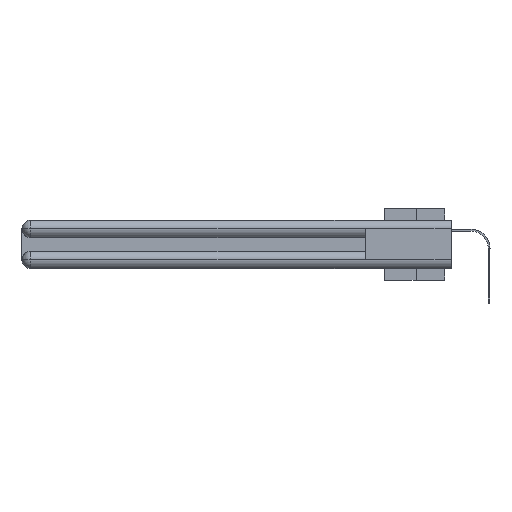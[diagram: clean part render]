
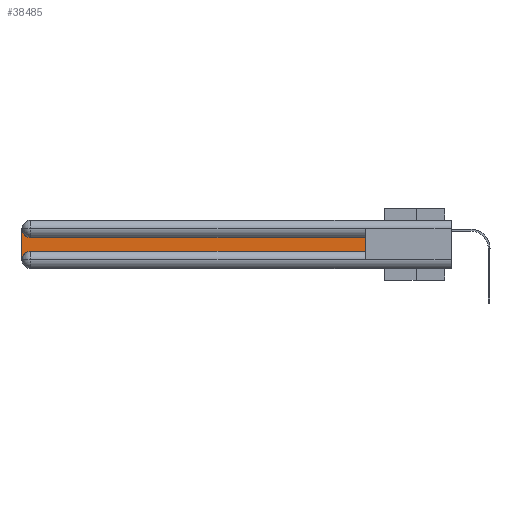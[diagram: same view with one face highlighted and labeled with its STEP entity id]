
A CAD part, left-side view. The second image highlights one B-rep face of the part: STEP entity #38485.
In plain terms, the highlighted planar face has unit normal (-1, 0, 0).
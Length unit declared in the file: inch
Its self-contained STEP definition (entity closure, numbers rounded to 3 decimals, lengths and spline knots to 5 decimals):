
#210 = DIRECTION ( 'NONE',  ( 1., 0., 0. ) ) ;
#868 = CARTESIAN_POINT ( 'NONE',  ( 0.075, 3., -0.0625 ) ) ;
#1109 = CARTESIAN_POINT ( 'NONE',  ( 0.075, 0.6, -0.2175 ) ) ;
#1456 = DIRECTION ( 'NONE',  ( 0., 0., 1. ) ) ;
#1462 = EDGE_CURVE ( 'NONE', #36980, #13549, #33551, .T. ) ;
#2479 = CARTESIAN_POINT ( 'NONE',  ( 0.075, 3., -0.2175 ) ) ;
#2937 = CARTESIAN_POINT ( 'NONE',  ( 0.075, 0.6, -0.1225 ) ) ;
#4326 = VECTOR ( 'NONE', #6533, 39.37008 ) ;
#5274 = ORIENTED_EDGE ( 'NONE', *, *, #5293, .T. ) ;
#5293 = EDGE_CURVE ( 'NONE', #35049, #37860, #30685, .T. ) ;
#5559 = LINE ( 'NONE', #17542, #23893 ) ;
#6024 = AXIS2_PLACEMENT_3D ( 'NONE', #17733, #10886, #17164 ) ;
#6533 = DIRECTION ( 'NONE',  ( 0., -1., 0. ) ) ;
#7232 = EDGE_CURVE ( 'NONE', #13549, #35049, #35408, .T. ) ;
#7799 = EDGE_CURVE ( 'NONE', #11284, #36980, #5559, .T. ) ;
#8370 = DIRECTION ( 'NONE',  ( 1., 0., 0. ) ) ;
#9089 = EDGE_CURVE ( 'NONE', #37860, #21161, #32810, .T. ) ;
#10886 = DIRECTION ( 'NONE',  ( 1., 0., 0. ) ) ;
#11266 = CARTESIAN_POINT ( 'NONE',  ( 0.075, 3., -0.2775 ) ) ;
#11284 = VERTEX_POINT ( 'NONE', #2937 ) ;
#11305 = FACE_OUTER_BOUND ( 'NONE', #34375, .T. ) ;
#13052 = ORIENTED_EDGE ( 'NONE', *, *, #7799, .T. ) ;
#13549 = VERTEX_POINT ( 'NONE', #868 ) ;
#13757 = EDGE_CURVE ( 'NONE', #21161, #11284, #31822, .T. ) ;
#14401 = DIRECTION ( 'NONE',  ( 0., 1., 0. ) ) ;
#15735 = VECTOR ( 'NONE', #35588, 39.37008 ) ;
#17164 = DIRECTION ( 'NONE',  ( 0., 0., -1. ) ) ;
#17542 = CARTESIAN_POINT ( 'NONE',  ( 0.075, 0.6, -0.1225 ) ) ;
#17733 = CARTESIAN_POINT ( 'NONE',  ( 0.075, 2.94, -0.0625 ) ) ;
#17892 = DIRECTION ( 'NONE',  ( 0., 0., -1. ) ) ;
#20025 = ORIENTED_EDGE ( 'NONE', *, *, #9089, .T. ) ;
#20145 = CARTESIAN_POINT ( 'NONE',  ( 0.075, 3., -0.1225 ) ) ;
#21021 = CARTESIAN_POINT ( 'NONE',  ( 0.075, 2.94, -0.2775 ) ) ;
#21161 = VERTEX_POINT ( 'NONE', #1109 ) ;
#22534 = AXIS2_PLACEMENT_3D ( 'NONE', #20145, #8370, #32276 ) ;
#22584 = AXIS2_PLACEMENT_3D ( 'NONE', #21021, #210, #17892 ) ;
#23149 = VECTOR ( 'NONE', #1456, 39.37008 ) ;
#23893 = VECTOR ( 'NONE', #14401, 39.37008 ) ;
#24774 = CARTESIAN_POINT ( 'NONE',  ( 0.075, 2.94, -0.2175 ) ) ;
#24956 = ORIENTED_EDGE ( 'NONE', *, *, #13757, .T. ) ;
#25368 = ORIENTED_EDGE ( 'NONE', *, *, #1462, .T. ) ;
#27106 = CARTESIAN_POINT ( 'NONE',  ( 0.075, 0.6, -0.2175 ) ) ;
#27643 = CARTESIAN_POINT ( 'NONE',  ( 0.075, 2.94, -0.1225 ) ) ;
#28300 = CARTESIAN_POINT ( 'NONE',  ( 0.075, 0.6, -0.2175 ) ) ;
#30685 = CIRCLE ( 'NONE', #22584, 0.06 ) ;
#31822 = LINE ( 'NONE', #28300, #23149 ) ;
#31971 = ORIENTED_EDGE ( 'NONE', *, *, #7232, .T. ) ;
#32276 = DIRECTION ( 'NONE',  ( 0., 0., -1. ) ) ;
#32810 = LINE ( 'NONE', #27106, #4326 ) ;
#33551 = CIRCLE ( 'NONE', #6024, 0.06 ) ;
#34375 = EDGE_LOOP ( 'NONE', ( #13052, #25368, #31971, #5274, #20025, #24956 ) ) ;
#35049 = VERTEX_POINT ( 'NONE', #11266 ) ;
#35408 = LINE ( 'NONE', #2479, #15735 ) ;
#35410 = PLANE ( 'NONE',  #22534 ) ;
#35588 = DIRECTION ( 'NONE',  ( 0., 0., -1. ) ) ;
#36980 = VERTEX_POINT ( 'NONE', #27643 ) ;
#37860 = VERTEX_POINT ( 'NONE', #24774 ) ;
#38485 = ADVANCED_FACE ( 'NONE', ( #11305 ), #35410, .F. ) ;
